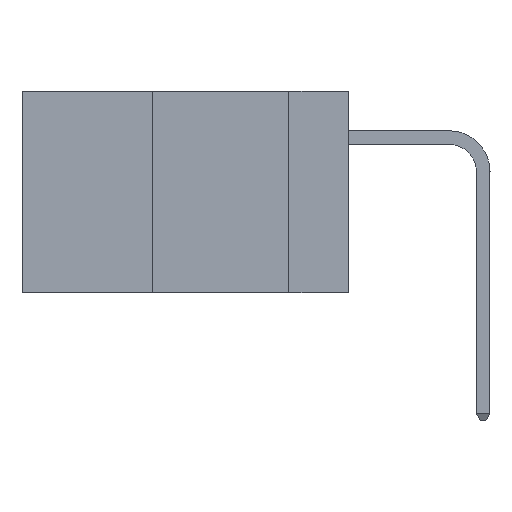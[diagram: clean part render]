
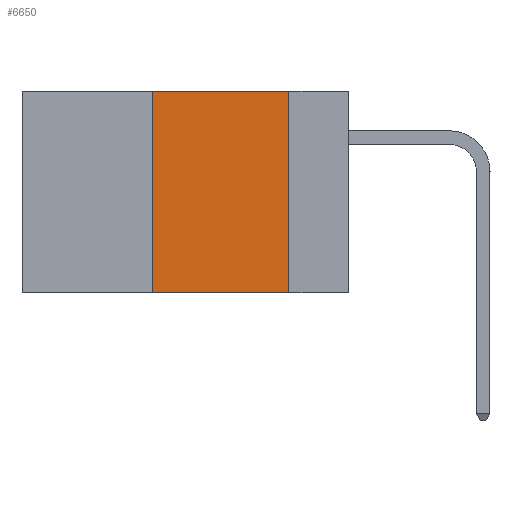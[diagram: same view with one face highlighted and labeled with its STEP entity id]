
A CAD part, left-side view. The second image highlights one B-rep face of the part: STEP entity #6650.
In plain terms, the highlighted planar face has unit normal (-1, 0, 0).
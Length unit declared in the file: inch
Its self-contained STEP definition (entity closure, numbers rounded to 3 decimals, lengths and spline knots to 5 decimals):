
#503 = PLANE ( 'NONE',  #11771 ) ;
#893 = CARTESIAN_POINT ( 'NONE',  ( 0., 0.36, 0. ) ) ;
#930 = CARTESIAN_POINT ( 'NONE',  ( 0., 0.11, 0. ) ) ;
#961 = VERTEX_POINT ( 'NONE', #13457 ) ;
#1085 = EDGE_CURVE ( 'NONE', #7509, #10924, #4190, .T. ) ;
#1595 = EDGE_CURVE ( 'NONE', #16382, #7509, #14209, .T. ) ;
#1784 = LINE ( 'NONE', #3175, #14703 ) ;
#1907 = DIRECTION ( 'NONE',  ( 1., 0., 0. ) ) ;
#3175 = CARTESIAN_POINT ( 'NONE',  ( 0., 0.6, -0.37 ) ) ;
#3661 = ORIENTED_EDGE ( 'NONE', *, *, #14256, .F. ) ;
#4190 = LINE ( 'NONE', #8549, #10466 ) ;
#4362 = VECTOR ( 'NONE', #15340, 39.37008 ) ;
#4382 = ORIENTED_EDGE ( 'NONE', *, *, #15647, .T. ) ;
#4501 = DIRECTION ( 'NONE',  ( 0., -1., 0. ) ) ;
#6650 = ADVANCED_FACE ( 'NONE', ( #9887 ), #503, .F. ) ;
#7509 = VERTEX_POINT ( 'NONE', #893 ) ;
#8161 = VECTOR ( 'NONE', #16124, 39.37008 ) ;
#8373 = ORIENTED_EDGE ( 'NONE', *, *, #1085, .F. ) ;
#8549 = CARTESIAN_POINT ( 'NONE',  ( 0., 0.6, 0. ) ) ;
#9587 = CARTESIAN_POINT ( 'NONE',  ( 0., 0.36, -0.37 ) ) ;
#9887 = FACE_OUTER_BOUND ( 'NONE', #16193, .T. ) ;
#10120 = CARTESIAN_POINT ( 'NONE',  ( 0., 0.11, 0. ) ) ;
#10466 = VECTOR ( 'NONE', #14191, 39.37008 ) ;
#10640 = ORIENTED_EDGE ( 'NONE', *, *, #1595, .F. ) ;
#10821 = DIRECTION ( 'NONE',  ( 0., 0., -1. ) ) ;
#10924 = VERTEX_POINT ( 'NONE', #930 ) ;
#11366 = LINE ( 'NONE', #10120, #8161 ) ;
#11771 = AXIS2_PLACEMENT_3D ( 'NONE', #14389, #1907, #10821 ) ;
#13457 = CARTESIAN_POINT ( 'NONE',  ( 0., 0.11, -0.37 ) ) ;
#14191 = DIRECTION ( 'NONE',  ( 0., -1., 0. ) ) ;
#14209 = LINE ( 'NONE', #16000, #4362 ) ;
#14256 = EDGE_CURVE ( 'NONE', #10924, #961, #11366, .T. ) ;
#14389 = CARTESIAN_POINT ( 'NONE',  ( 0., 0.6, 0. ) ) ;
#14703 = VECTOR ( 'NONE', #4501, 39.37008 ) ;
#15340 = DIRECTION ( 'NONE',  ( 0., 0., 1. ) ) ;
#15647 = EDGE_CURVE ( 'NONE', #16382, #961, #1784, .T. ) ;
#16000 = CARTESIAN_POINT ( 'NONE',  ( 0., 0.36, 0. ) ) ;
#16124 = DIRECTION ( 'NONE',  ( 0., 0., -1. ) ) ;
#16193 = EDGE_LOOP ( 'NONE', ( #3661, #8373, #10640, #4382 ) ) ;
#16382 = VERTEX_POINT ( 'NONE', #9587 ) ;
